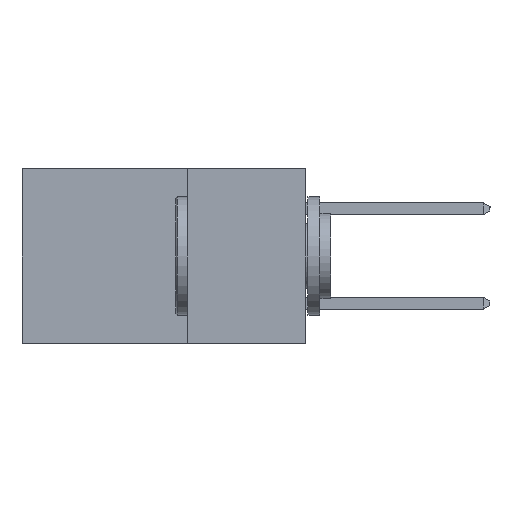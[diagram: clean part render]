
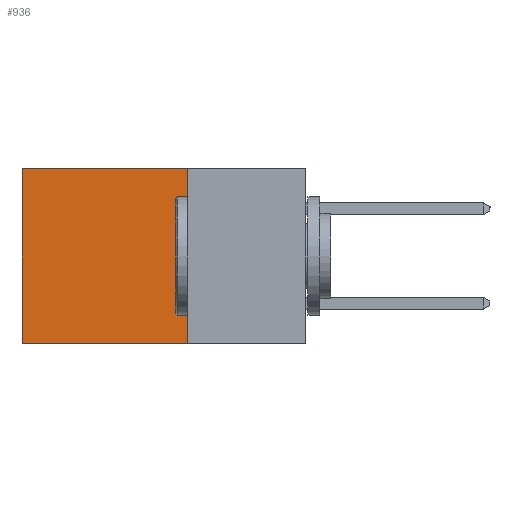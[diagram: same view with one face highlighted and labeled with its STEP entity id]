
A CAD part, left-side view. The second image highlights one B-rep face of the part: STEP entity #936.
In plain terms, the highlighted planar face has unit normal (-1, 0, 0).
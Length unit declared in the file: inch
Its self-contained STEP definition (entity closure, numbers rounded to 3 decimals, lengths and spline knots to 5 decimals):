
#45 = EDGE_CURVE ( 'NONE', #1313, #1547, #4830, .T. ) ;
#232 = CARTESIAN_POINT ( 'NONE',  ( 0.2615, 0.25, -0.37 ) ) ;
#445 = CARTESIAN_POINT ( 'NONE',  ( 0.2615, 0.25, -0.37 ) ) ;
#693 = CARTESIAN_POINT ( 'NONE',  ( 0.2615, 0.25, 0. ) ) ;
#822 = CARTESIAN_POINT ( 'NONE',  ( 0.2615, 0.6, -0.37 ) ) ;
#861 = ORIENTED_EDGE ( 'NONE', *, *, #45, .F. ) ;
#936 = ADVANCED_FACE ( 'NONE', ( #3117 ), #8732, .F. ) ;
#1251 = EDGE_LOOP ( 'NONE', ( #8584, #861, #7673, #3500 ) ) ;
#1284 = CARTESIAN_POINT ( 'NONE',  ( 0.2615, 0.25, -0.37 ) ) ;
#1313 = VERTEX_POINT ( 'NONE', #1284 ) ;
#1547 = VERTEX_POINT ( 'NONE', #11509 ) ;
#1595 = LINE ( 'NONE', #693, #6228 ) ;
#2195 = DIRECTION ( 'NONE',  ( 0., 0., -1. ) ) ;
#2558 = AXIS2_PLACEMENT_3D ( 'NONE', #445, #4110, #4937 ) ;
#2695 = CARTESIAN_POINT ( 'NONE',  ( 0.2615, 0.25, 0. ) ) ;
#3090 = LINE ( 'NONE', #232, #8989 ) ;
#3117 = FACE_OUTER_BOUND ( 'NONE', #1251, .T. ) ;
#3121 = DIRECTION ( 'NONE',  ( 0., 1., 0. ) ) ;
#3236 = VECTOR ( 'NONE', #5362, 39.37008 ) ;
#3253 = VERTEX_POINT ( 'NONE', #4976 ) ;
#3500 = ORIENTED_EDGE ( 'NONE', *, *, #4473, .T. ) ;
#4110 = DIRECTION ( 'NONE',  ( 1., 0., 0. ) ) ;
#4362 = DIRECTION ( 'NONE',  ( 0., 1., 0. ) ) ;
#4473 = EDGE_CURVE ( 'NONE', #7238, #3253, #1595, .T. ) ;
#4830 = LINE ( 'NONE', #5886, #11273 ) ;
#4937 = DIRECTION ( 'NONE',  ( 0., 0., -1. ) ) ;
#4976 = CARTESIAN_POINT ( 'NONE',  ( 0.2615, 0.6, 0. ) ) ;
#5362 = DIRECTION ( 'NONE',  ( 0., 0., -1. ) ) ;
#5886 = CARTESIAN_POINT ( 'NONE',  ( 0.2615, 0.25, -0.37 ) ) ;
#6228 = VECTOR ( 'NONE', #4362, 39.37008 ) ;
#7238 = VERTEX_POINT ( 'NONE', #2695 ) ;
#7673 = ORIENTED_EDGE ( 'NONE', *, *, #9604, .F. ) ;
#8389 = EDGE_CURVE ( 'NONE', #3253, #1547, #8915, .T. ) ;
#8584 = ORIENTED_EDGE ( 'NONE', *, *, #8389, .T. ) ;
#8732 = PLANE ( 'NONE',  #2558 ) ;
#8915 = LINE ( 'NONE', #822, #3236 ) ;
#8989 = VECTOR ( 'NONE', #2195, 39.37008 ) ;
#9604 = EDGE_CURVE ( 'NONE', #7238, #1313, #3090, .T. ) ;
#11273 = VECTOR ( 'NONE', #3121, 39.37008 ) ;
#11509 = CARTESIAN_POINT ( 'NONE',  ( 0.2615, 0.6, -0.37 ) ) ;
